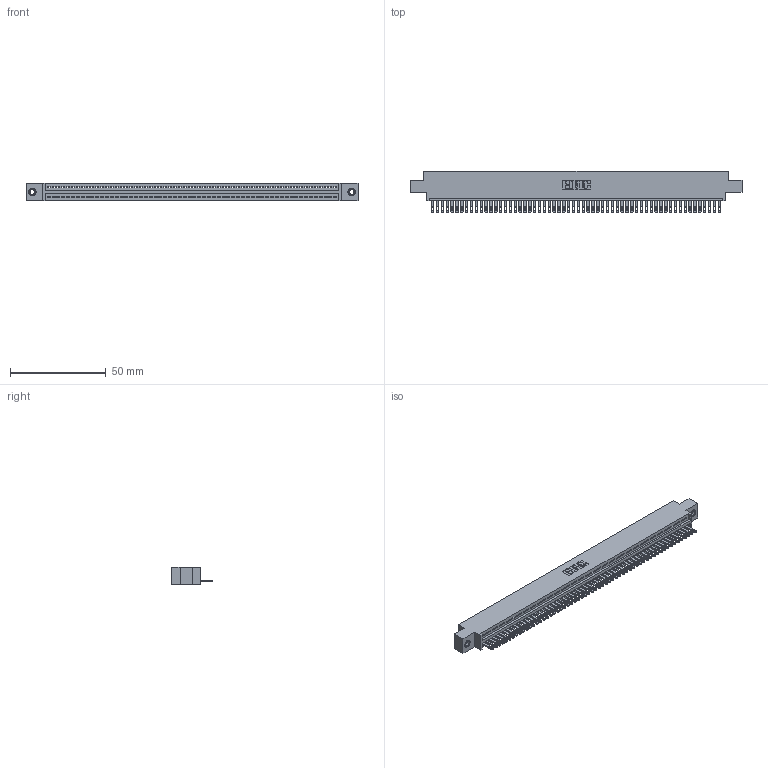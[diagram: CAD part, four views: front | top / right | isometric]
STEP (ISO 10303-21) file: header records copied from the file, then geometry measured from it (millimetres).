
FILE_DESCRIPTION (( 'STEP AP203' ), '1' );
FILE_NAME ('895-060-500-607.STEP', '2020-09-28T05:03:37', ( '' ), ( '' ), 'SwSTEP 2.0', 'SolidWorks 2020', '' );
FILE_SCHEMA (( 'CONFIG_CONTROL_DESIGN' ));
Length unit declared in the file: inch
Products named in the file (4): 845 Part_0.170 Offset - 0.156 Dia-TI; 345-250-001_345-250-005-103; 345-292-001_345-293-100; 895-060-500-607
Assembly tree (63 placements, depth 2):
  895-060-500-607
    845 Part_0.170 Offset - 0.156 Dia-TI
    345-292-001_345-293-100  x60
    345-250-001_345-250-005-103  x2
Bounding box: 173.61 x 21.51 x 9.4 mm (x, y, z)
Volume: 16547.2 mm3; surface area: 22528.3 mm2
Topology: 63 solids, 63 shells, 3430 faces, 10569 edges, 7038 vertices
Faces by surface type: plane 2156, cylinder 1258, cone 12, torus 4
Entity records: 43982 total; most frequent: CARTESIAN_POINT 7599, ORIENTED_EDGE 7586, DIRECTION 6639, EDGE_CURVE 3793, VECTOR 3397, LINE 3397, VERTEX_POINT 2524, AXIS2_PLACEMENT_3D 1621
